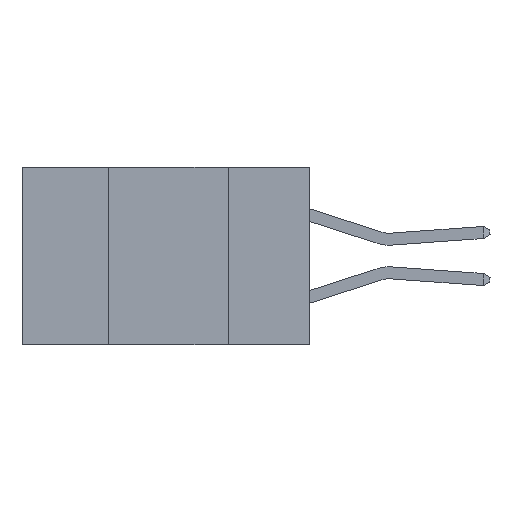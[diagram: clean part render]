
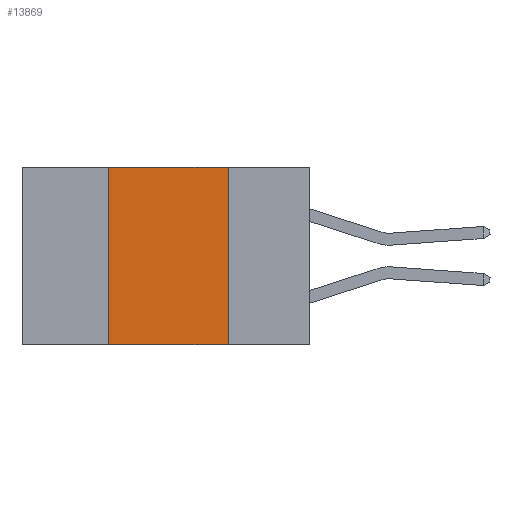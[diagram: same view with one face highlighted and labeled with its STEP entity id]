
A CAD part, left-side view. The second image highlights one B-rep face of the part: STEP entity #13869.
In plain terms, the highlighted planar face has unit normal (-1, 0, 0).
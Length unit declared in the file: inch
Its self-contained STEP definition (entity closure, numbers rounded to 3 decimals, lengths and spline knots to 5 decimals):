
#1457 = LINE ( 'NONE', #10981, #15495 ) ;
#1658 = CARTESIAN_POINT ( 'NONE',  ( 0., 0.42, -0.37 ) ) ;
#2518 = ORIENTED_EDGE ( 'NONE', *, *, #9861, .F. ) ;
#2901 = CARTESIAN_POINT ( 'NONE',  ( 0., 0.42, 0. ) ) ;
#3715 = VERTEX_POINT ( 'NONE', #11524 ) ;
#3874 = ORIENTED_EDGE ( 'NONE', *, *, #11126, .T. ) ;
#5100 = CARTESIAN_POINT ( 'NONE',  ( 0., 0.6, 0. ) ) ;
#5284 = VECTOR ( 'NONE', #13937, 39.37008 ) ;
#6036 = VERTEX_POINT ( 'NONE', #8409 ) ;
#6231 = DIRECTION ( 'NONE',  ( 0., -1., 0. ) ) ;
#6236 = EDGE_CURVE ( 'NONE', #12027, #3715, #1457, .T. ) ;
#6967 = DIRECTION ( 'NONE',  ( 0., -1., 0. ) ) ;
#6975 = VECTOR ( 'NONE', #6231, 39.37008 ) ;
#7406 = EDGE_LOOP ( 'NONE', ( #13407, #2518, #9492, #3874 ) ) ;
#7968 = CARTESIAN_POINT ( 'NONE',  ( 0., 0.6, 0. ) ) ;
#8409 = CARTESIAN_POINT ( 'NONE',  ( 0., 0.42, 0. ) ) ;
#9175 = PLANE ( 'NONE',  #12791 ) ;
#9492 = ORIENTED_EDGE ( 'NONE', *, *, #15256, .F. ) ;
#9861 = EDGE_CURVE ( 'NONE', #6036, #12027, #13464, .T. ) ;
#10098 = CARTESIAN_POINT ( 'NONE',  ( 0., 0.17, 0. ) ) ;
#10429 = LINE ( 'NONE', #2901, #5284 ) ;
#10558 = VERTEX_POINT ( 'NONE', #1658 ) ;
#10981 = CARTESIAN_POINT ( 'NONE',  ( 0., 0.17, 0. ) ) ;
#11126 = EDGE_CURVE ( 'NONE', #10558, #3715, #14577, .T. ) ;
#11524 = CARTESIAN_POINT ( 'NONE',  ( 0., 0.17, -0.37 ) ) ;
#12027 = VERTEX_POINT ( 'NONE', #10098 ) ;
#12093 = VECTOR ( 'NONE', #6967, 39.37008 ) ;
#12226 = DIRECTION ( 'NONE',  ( 0., 0., -1. ) ) ;
#12371 = FACE_OUTER_BOUND ( 'NONE', #7406, .T. ) ;
#12791 = AXIS2_PLACEMENT_3D ( 'NONE', #7968, #12838, #15308 ) ;
#12838 = DIRECTION ( 'NONE',  ( 1., 0., 0. ) ) ;
#13407 = ORIENTED_EDGE ( 'NONE', *, *, #6236, .F. ) ;
#13464 = LINE ( 'NONE', #5100, #6975 ) ;
#13869 = ADVANCED_FACE ( 'NONE', ( #12371 ), #9175, .F. ) ;
#13937 = DIRECTION ( 'NONE',  ( 0., 0., 1. ) ) ;
#14070 = CARTESIAN_POINT ( 'NONE',  ( 0., 0.6, -0.37 ) ) ;
#14577 = LINE ( 'NONE', #14070, #12093 ) ;
#15256 = EDGE_CURVE ( 'NONE', #10558, #6036, #10429, .T. ) ;
#15308 = DIRECTION ( 'NONE',  ( 0., 0., -1. ) ) ;
#15495 = VECTOR ( 'NONE', #12226, 39.37008 ) ;
